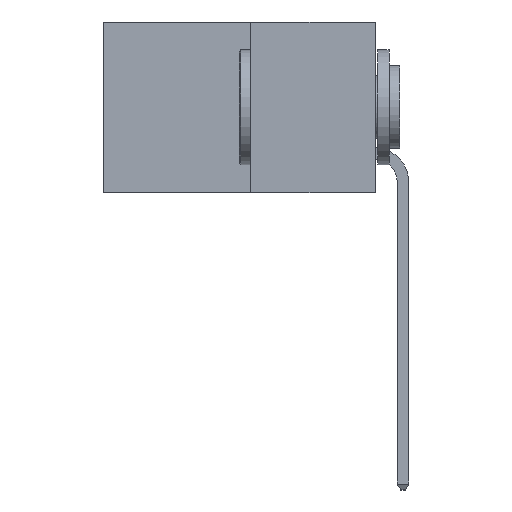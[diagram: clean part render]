
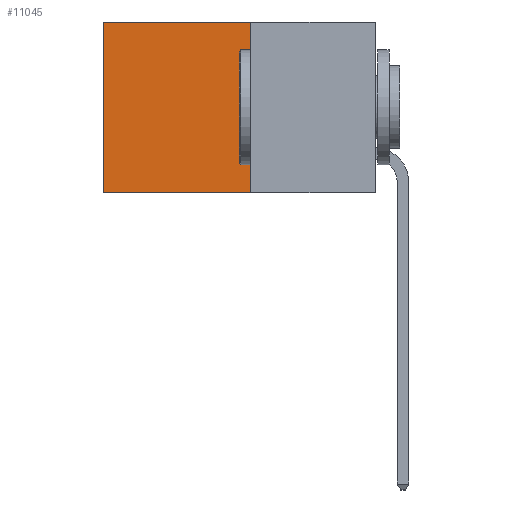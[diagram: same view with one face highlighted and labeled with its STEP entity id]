
A CAD part, left-side view. The second image highlights one B-rep face of the part: STEP entity #11045.
In plain terms, the highlighted planar face has unit normal (-1, 0, 0).
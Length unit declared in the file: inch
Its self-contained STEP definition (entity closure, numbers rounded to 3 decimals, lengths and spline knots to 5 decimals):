
#98 = ORIENTED_EDGE ( 'NONE', *, *, #11728, .T. ) ;
#158 = ORIENTED_EDGE ( 'NONE', *, *, #6111, .F. ) ;
#242 = ORIENTED_EDGE ( 'NONE', *, *, #839, .F. ) ;
#338 = ORIENTED_EDGE ( 'NONE', *, *, #6143, .T. ) ;
#725 = VERTEX_POINT ( 'NONE', #6878 ) ;
#839 = EDGE_CURVE ( 'NONE', #7805, #8073, #8469, .T. ) ;
#991 = CARTESIAN_POINT ( 'NONE',  ( 0.277, 0.27, -0.37 ) ) ;
#2096 = LINE ( 'NONE', #11556, #7629 ) ;
#2149 = AXIS2_PLACEMENT_3D ( 'NONE', #10930, #4809, #11929 ) ;
#2620 = EDGE_LOOP ( 'NONE', ( #98, #158, #242, #338 ) ) ;
#3341 = VERTEX_POINT ( 'NONE', #10733 ) ;
#3736 = PLANE ( 'NONE',  #2149 ) ;
#4232 = VECTOR ( 'NONE', #11315, 39.37008 ) ;
#4809 = DIRECTION ( 'NONE',  ( 1., 0., 0. ) ) ;
#5986 = CARTESIAN_POINT ( 'NONE',  ( 0.277, 0.59, -0.37 ) ) ;
#6111 = EDGE_CURVE ( 'NONE', #8073, #3341, #2096, .T. ) ;
#6143 = EDGE_CURVE ( 'NONE', #7805, #725, #7312, .T. ) ;
#6160 = CARTESIAN_POINT ( 'NONE',  ( 0.277, 0.27, -0.37 ) ) ;
#6732 = FACE_OUTER_BOUND ( 'NONE', #2620, .T. ) ;
#6878 = CARTESIAN_POINT ( 'NONE',  ( 0.277, 0.59, 0. ) ) ;
#6986 = DIRECTION ( 'NONE',  ( 0., 0., -1. ) ) ;
#7312 = LINE ( 'NONE', #11384, #4232 ) ;
#7629 = VECTOR ( 'NONE', #11540, 39.37008 ) ;
#7636 = LINE ( 'NONE', #5986, #10019 ) ;
#7805 = VERTEX_POINT ( 'NONE', #11613 ) ;
#7840 = VECTOR ( 'NONE', #9453, 39.37008 ) ;
#8073 = VERTEX_POINT ( 'NONE', #6160 ) ;
#8469 = LINE ( 'NONE', #991, #7840 ) ;
#9453 = DIRECTION ( 'NONE',  ( 0., 0., -1. ) ) ;
#10019 = VECTOR ( 'NONE', #6986, 39.37008 ) ;
#10733 = CARTESIAN_POINT ( 'NONE',  ( 0.277, 0.59, -0.37 ) ) ;
#10930 = CARTESIAN_POINT ( 'NONE',  ( 0.277, 0.27, -0.37 ) ) ;
#11045 = ADVANCED_FACE ( 'NONE', ( #6732 ), #3736, .F. ) ;
#11315 = DIRECTION ( 'NONE',  ( 0., 1., 0. ) ) ;
#11384 = CARTESIAN_POINT ( 'NONE',  ( 0.277, 0.27, 0. ) ) ;
#11540 = DIRECTION ( 'NONE',  ( 0., 1., 0. ) ) ;
#11556 = CARTESIAN_POINT ( 'NONE',  ( 0.277, 0.27, -0.37 ) ) ;
#11613 = CARTESIAN_POINT ( 'NONE',  ( 0.277, 0.27, 0. ) ) ;
#11728 = EDGE_CURVE ( 'NONE', #725, #3341, #7636, .T. ) ;
#11929 = DIRECTION ( 'NONE',  ( 0., 0., -1. ) ) ;
